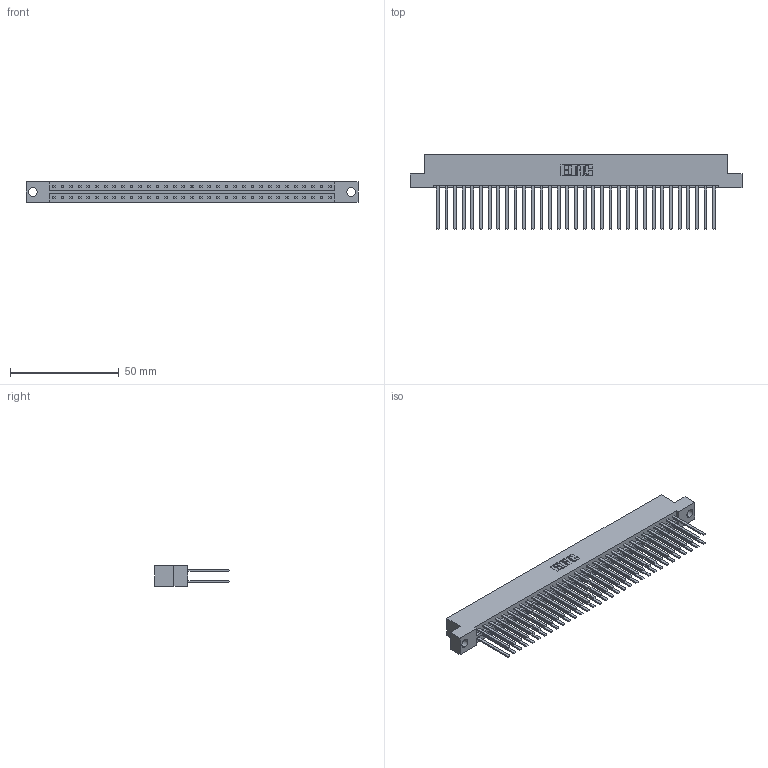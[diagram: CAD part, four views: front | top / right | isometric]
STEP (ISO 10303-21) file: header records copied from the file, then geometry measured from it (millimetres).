
FILE_DESCRIPTION (( 'STEP AP203' ), '1' );
FILE_NAME ('333-066-544-204.STEP', '2018-08-04T11:40:23', ( '' ), ( '' ), 'SwSTEP 2.0', 'SolidWorks 2016', '' );
FILE_SCHEMA (( 'CONFIG_CONTROL_DESIGN' ));
Length unit declared in the file: inch
Products named in the file (3): 333-066-544-204; 333 Part_Flush - .156 Dia - TH; 345-292-001_345-293-144
Assembly tree (67 placements, depth 2):
  333-066-544-204
    333 Part_Flush - .156 Dia - TH
    345-292-001_345-293-144  x66
Bounding box: 152.3 x 34.3 x 9.4 mm (x, y, z)
Volume: 16302 mm3; surface area: 21954.6 mm2
Topology: 67 solids, 67 shells, 3150 faces, 9353 edges, 6146 vertices
Faces by surface type: plane 2182, cylinder 968
Entity records: 22213 total; most frequent: CARTESIAN_POINT 3690, ORIENTED_EDGE 3626, DIRECTION 3165, EDGE_CURVE 1813, LINE 1689, VECTOR 1689, VERTEX_POINT 1206, AXIS2_PLACEMENT_3D 738
